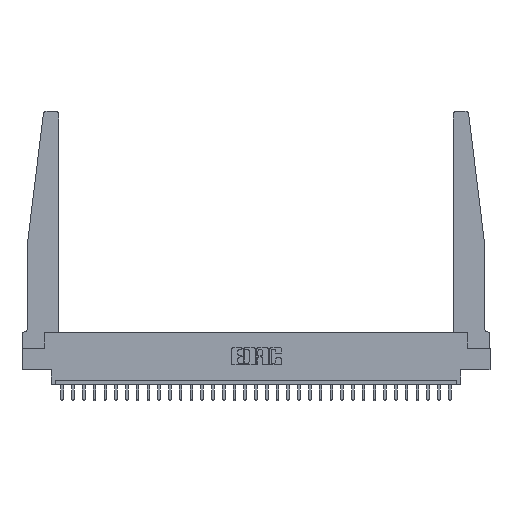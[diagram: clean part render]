
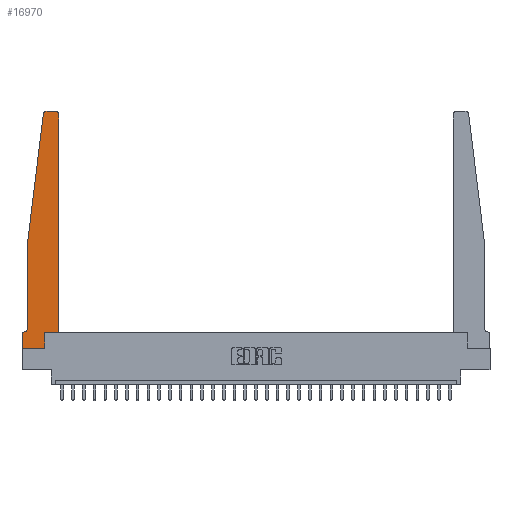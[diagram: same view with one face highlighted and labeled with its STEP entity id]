
A CAD part, top view. The second image highlights one B-rep face of the part: STEP entity #16970.
In plain terms, the highlighted planar face has unit normal (0, 0, 1).
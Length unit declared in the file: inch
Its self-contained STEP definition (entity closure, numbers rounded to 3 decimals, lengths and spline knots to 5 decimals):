
#579 = DIRECTION ( 'NONE',  ( 0., 0., 1. ) ) ;
#593 = DIRECTION ( 'NONE',  ( 1., 0., 0. ) ) ;
#1363 = DIRECTION ( 'NONE',  ( 0., -1., 0. ) ) ;
#1717 = ORIENTED_EDGE ( 'NONE', *, *, #12355, .T. ) ;
#1743 = VECTOR ( 'NONE', #20585, 39.37008 ) ;
#1753 = VECTOR ( 'NONE', #24664, 39.37008 ) ;
#1974 = CARTESIAN_POINT ( 'NONE',  ( 0.065, 0.1875, 0.37 ) ) ;
#2436 = EDGE_CURVE ( 'NONE', #10299, #9389, #14768, .T. ) ;
#2564 = DIRECTION ( 'NONE',  ( -1., 0., 0. ) ) ;
#2673 = VERTEX_POINT ( 'NONE', #14591 ) ;
#2959 = VERTEX_POINT ( 'NONE', #6158 ) ;
#3182 = DIRECTION ( 'NONE',  ( 0., 0., 1. ) ) ;
#3455 = CARTESIAN_POINT ( 'NONE',  ( 0.065, 1.25, 0.37 ) ) ;
#4229 = EDGE_CURVE ( 'NONE', #6906, #8418, #11023, .T. ) ;
#5140 = VECTOR ( 'NONE', #9952, 39.37008 ) ;
#5406 = VECTOR ( 'NONE', #1363, 39.37008 ) ;
#5586 = AXIS2_PLACEMENT_3D ( 'NONE', #16849, #3182, #18921 ) ;
#6158 = CARTESIAN_POINT ( 'NONE',  ( 0.24675, 2.72367, 0.37 ) ) ;
#6582 = LINE ( 'NONE', #1974, #26246 ) ;
#6799 = AXIS2_PLACEMENT_3D ( 'NONE', #18234, #25337, #593 ) ;
#6901 = ORIENTED_EDGE ( 'NONE', *, *, #19206, .T. ) ;
#6906 = VERTEX_POINT ( 'NONE', #8609 ) ;
#7018 = CARTESIAN_POINT ( 'NONE',  ( 0.015, 0.1875, 0.37 ) ) ;
#7067 = LINE ( 'NONE', #20297, #24790 ) ;
#7193 = ORIENTED_EDGE ( 'NONE', *, *, #16462, .T. ) ;
#8073 = EDGE_CURVE ( 'NONE', #2959, #10299, #16552, .T. ) ;
#8418 = VERTEX_POINT ( 'NONE', #23249 ) ;
#8502 = VECTOR ( 'NONE', #12988, 39.37008 ) ;
#8609 = CARTESIAN_POINT ( 'NONE',  ( 0.395, 2.75, 0.37 ) ) ;
#8670 = ORIENTED_EDGE ( 'NONE', *, *, #9630, .T. ) ;
#8935 = ORIENTED_EDGE ( 'NONE', *, *, #8073, .T. ) ;
#8973 = ORIENTED_EDGE ( 'NONE', *, *, #2436, .T. ) ;
#9389 = VERTEX_POINT ( 'NONE', #15254 ) ;
#9630 = EDGE_CURVE ( 'NONE', #22405, #11026, #28639, .T. ) ;
#9945 = CIRCLE ( 'NONE', #16061, 0.03 ) ;
#9952 = DIRECTION ( 'NONE',  ( -0.122, -0.992, 0. ) ) ;
#10156 = LINE ( 'NONE', #24021, #13877 ) ;
#10299 = VERTEX_POINT ( 'NONE', #3455 ) ;
#10896 = ORIENTED_EDGE ( 'NONE', *, *, #20711, .T. ) ;
#11023 = LINE ( 'NONE', #11180, #11568 ) ;
#11026 = VERTEX_POINT ( 'NONE', #14238 ) ;
#11180 = CARTESIAN_POINT ( 'NONE',  ( 0.25, 2.75, 0.37 ) ) ;
#11352 = EDGE_LOOP ( 'NONE', ( #24111, #7193, #8935, #8973, #12735, #1717, #6901, #10896, #11806, #8670, #25212, #25588 ) ) ;
#11568 = VECTOR ( 'NONE', #13514, 39.37008 ) ;
#11606 = FACE_OUTER_BOUND ( 'NONE', #11352, .T. ) ;
#11806 = ORIENTED_EDGE ( 'NONE', *, *, #12346, .T. ) ;
#12346 = EDGE_CURVE ( 'NONE', #2673, #22405, #15217, .T. ) ;
#12355 = EDGE_CURVE ( 'NONE', #25174, #13568, #6582, .T. ) ;
#12735 = ORIENTED_EDGE ( 'NONE', *, *, #13313, .T. ) ;
#12988 = DIRECTION ( 'NONE',  ( 1., 0., 0. ) ) ;
#13313 = EDGE_CURVE ( 'NONE', #9389, #25174, #29068, .T. ) ;
#13335 = DIRECTION ( 'NONE',  ( 1., 0., 0. ) ) ;
#13514 = DIRECTION ( 'NONE',  ( -1., 0., 0. ) ) ;
#13568 = VERTEX_POINT ( 'NONE', #27427 ) ;
#13606 = DIRECTION ( 'NONE',  ( 0., 1., 0. ) ) ;
#13877 = VECTOR ( 'NONE', #23578, 39.37008 ) ;
#14238 = CARTESIAN_POINT ( 'NONE',  ( 0.425, 0.18, 0.37 ) ) ;
#14591 = CARTESIAN_POINT ( 'NONE',  ( 0.2605, 0., 0.37 ) ) ;
#14768 = LINE ( 'NONE', #21816, #5406 ) ;
#15217 = LINE ( 'NONE', #18021, #1753 ) ;
#15254 = CARTESIAN_POINT ( 'NONE',  ( 0.065, 0.2375, 0.37 ) ) ;
#16061 = AXIS2_PLACEMENT_3D ( 'NONE', #24723, #579, #13335 ) ;
#16462 = EDGE_CURVE ( 'NONE', #8418, #2959, #27188, .T. ) ;
#16552 = LINE ( 'NONE', #21134, #5140 ) ;
#16849 = CARTESIAN_POINT ( 'NONE',  ( 0.27653, 2.72, 0.37 ) ) ;
#16970 = ADVANCED_FACE ( 'NONE', ( #11606 ), #20758, .T. ) ;
#17391 = DIRECTION ( 'NONE',  ( -1., 0., 0. ) ) ;
#17778 = CARTESIAN_POINT ( 'NONE',  ( 0., 0., 0.37 ) ) ;
#18021 = CARTESIAN_POINT ( 'NONE',  ( 0.2605, 0.18, 0.37 ) ) ;
#18234 = CARTESIAN_POINT ( 'NONE',  ( 0., 0.1875, 0.37 ) ) ;
#18921 = DIRECTION ( 'NONE',  ( 1., 0., 0. ) ) ;
#19206 = EDGE_CURVE ( 'NONE', #13568, #21422, #10156, .T. ) ;
#20066 = EDGE_CURVE ( 'NONE', #11026, #28517, #7067, .T. ) ;
#20297 = CARTESIAN_POINT ( 'NONE',  ( 0.425, 0.18, 0.37 ) ) ;
#20585 = DIRECTION ( 'NONE',  ( 1., 0., 0. ) ) ;
#20711 = EDGE_CURVE ( 'NONE', #21422, #2673, #24588, .T. ) ;
#20758 = PLANE ( 'NONE',  #6799 ) ;
#21106 = CARTESIAN_POINT ( 'NONE',  ( 0.425, 2.72, 0.37 ) ) ;
#21134 = CARTESIAN_POINT ( 'NONE',  ( 0.065, 1.25, 0.37 ) ) ;
#21422 = VERTEX_POINT ( 'NONE', #26253 ) ;
#21816 = CARTESIAN_POINT ( 'NONE',  ( 0.065, 1.25, 0.37 ) ) ;
#22405 = VERTEX_POINT ( 'NONE', #27933 ) ;
#23249 = CARTESIAN_POINT ( 'NONE',  ( 0.27653, 2.75, 0.37 ) ) ;
#23578 = DIRECTION ( 'NONE',  ( 0., -1., 0. ) ) ;
#24021 = CARTESIAN_POINT ( 'NONE',  ( 0., 0., 0.37 ) ) ;
#24111 = ORIENTED_EDGE ( 'NONE', *, *, #4229, .T. ) ;
#24240 = CARTESIAN_POINT ( 'NONE',  ( 0.425, 0.18, 0.37 ) ) ;
#24588 = LINE ( 'NONE', #17778, #1743 ) ;
#24664 = DIRECTION ( 'NONE',  ( 0., 1., 0. ) ) ;
#24723 = CARTESIAN_POINT ( 'NONE',  ( 0.395, 2.72, 0.37 ) ) ;
#24790 = VECTOR ( 'NONE', #13606, 39.37008 ) ;
#25174 = VERTEX_POINT ( 'NONE', #7018 ) ;
#25212 = ORIENTED_EDGE ( 'NONE', *, *, #20066, .T. ) ;
#25337 = DIRECTION ( 'NONE',  ( 0., 0., 1. ) ) ;
#25588 = ORIENTED_EDGE ( 'NONE', *, *, #27632, .T. ) ;
#26246 = VECTOR ( 'NONE', #2564, 39.37008 ) ;
#26253 = CARTESIAN_POINT ( 'NONE',  ( 0., 0., 0.37 ) ) ;
#26536 = DIRECTION ( 'NONE',  ( 0., 0., -1. ) ) ;
#27188 = CIRCLE ( 'NONE', #5586, 0.03 ) ;
#27427 = CARTESIAN_POINT ( 'NONE',  ( 0., 0.1875, 0.37 ) ) ;
#27632 = EDGE_CURVE ( 'NONE', #28517, #6906, #9945, .T. ) ;
#27933 = CARTESIAN_POINT ( 'NONE',  ( 0.2605, 0.18, 0.37 ) ) ;
#28328 = CARTESIAN_POINT ( 'NONE',  ( 0.015, 0.2375, 0.37 ) ) ;
#28517 = VERTEX_POINT ( 'NONE', #21106 ) ;
#28570 = AXIS2_PLACEMENT_3D ( 'NONE', #28328, #26536, #17391 ) ;
#28639 = LINE ( 'NONE', #24240, #8502 ) ;
#29068 = CIRCLE ( 'NONE', #28570, 0.05 ) ;
